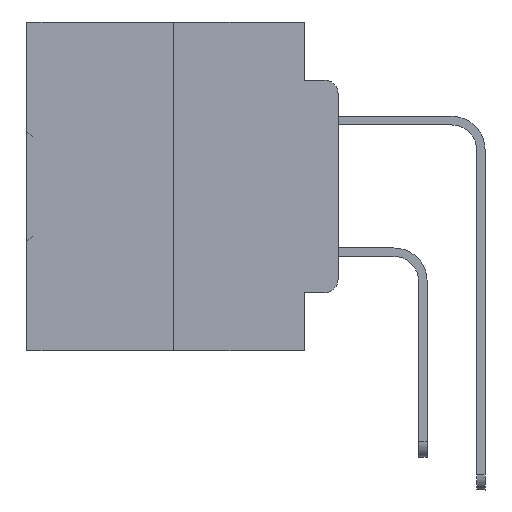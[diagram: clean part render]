
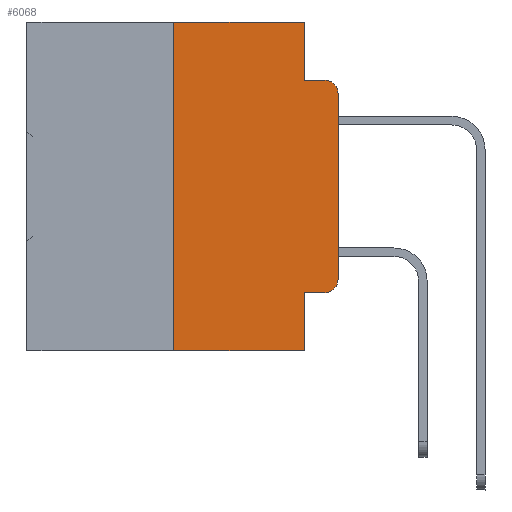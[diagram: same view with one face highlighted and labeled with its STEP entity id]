
A CAD part, left-side view. The second image highlights one B-rep face of the part: STEP entity #6068.
In plain terms, the highlighted planar face has unit normal (-1, 0, 0).
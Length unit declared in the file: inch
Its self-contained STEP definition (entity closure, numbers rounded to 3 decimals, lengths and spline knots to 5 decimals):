
#36 = ORIENTED_EDGE ( 'NONE', *, *, #22810, .F. ) ;
#89 = VECTOR ( 'NONE', #27309, 39.37008 ) ;
#466 = ORIENTED_EDGE ( 'NONE', *, *, #15825, .T. ) ;
#663 = DIRECTION ( 'NONE',  ( 0., -1., 0. ) ) ;
#906 = DIRECTION ( 'NONE',  ( 0., 0., 1. ) ) ;
#1231 = VERTEX_POINT ( 'NONE', #10744 ) ;
#1552 = CIRCLE ( 'NONE', #6538, 0.02 ) ;
#1707 = DIRECTION ( 'NONE',  ( 0., -1., 0. ) ) ;
#2793 = PLANE ( 'NONE',  #28297 ) ;
#3289 = VERTEX_POINT ( 'NONE', #22369 ) ;
#3346 = VERTEX_POINT ( 'NONE', #16937 ) ;
#3706 = EDGE_CURVE ( 'NONE', #19397, #1231, #22137, .T. ) ;
#4393 = CARTESIAN_POINT ( 'NONE',  ( 0., 0., -0.1085 ) ) ;
#5710 = DIRECTION ( 'NONE',  ( 0., 0., -1. ) ) ;
#6043 = EDGE_CURVE ( 'NONE', #19520, #1231, #1552, .T. ) ;
#6068 = ADVANCED_FACE ( 'NONE', ( #23015 ), #2793, .F. ) ;
#6453 = CARTESIAN_POINT ( 'NONE',  ( 0., 0.051, 0. ) ) ;
#6538 = AXIS2_PLACEMENT_3D ( 'NONE', #23588, #22820, #5710 ) ;
#6706 = AXIS2_PLACEMENT_3D ( 'NONE', #33310, #6827, #21218 ) ;
#6827 = DIRECTION ( 'NONE',  ( -1., 0., 0. ) ) ;
#6856 = LINE ( 'NONE', #18724, #20989 ) ;
#6894 = EDGE_LOOP ( 'NONE', ( #20061, #29721, #15955, #14135, #18119, #36357, #16792, #36, #466, #9473 ) ) ;
#7526 = LINE ( 'NONE', #15896, #27711 ) ;
#8056 = CARTESIAN_POINT ( 'NONE',  ( 0., 0.473, 0. ) ) ;
#8742 = VECTOR ( 'NONE', #31503, 39.37008 ) ;
#9473 = ORIENTED_EDGE ( 'NONE', *, *, #30266, .T. ) ;
#10744 = CARTESIAN_POINT ( 'NONE',  ( 0., 0.02, -0.0885 ) ) ;
#12270 = LINE ( 'NONE', #6453, #15726 ) ;
#12932 = CARTESIAN_POINT ( 'NONE',  ( 0., 0., -0.3915 ) ) ;
#13341 = VECTOR ( 'NONE', #663, 39.37008 ) ;
#14075 = DIRECTION ( 'NONE',  ( 1., 0., 0. ) ) ;
#14135 = ORIENTED_EDGE ( 'NONE', *, *, #27600, .F. ) ;
#15726 = VECTOR ( 'NONE', #17947, 39.37008 ) ;
#15825 = EDGE_CURVE ( 'NONE', #3289, #36625, #21860, .T. ) ;
#15896 = CARTESIAN_POINT ( 'NONE',  ( 0., 0., 0. ) ) ;
#15955 = ORIENTED_EDGE ( 'NONE', *, *, #3706, .F. ) ;
#16101 = CARTESIAN_POINT ( 'NONE',  ( 0., 0.051, 0. ) ) ;
#16626 = EDGE_CURVE ( 'NONE', #20588, #19520, #7526, .T. ) ;
#16792 = ORIENTED_EDGE ( 'NONE', *, *, #18825, .T. ) ;
#16937 = CARTESIAN_POINT ( 'NONE',  ( 0., 0.25, -0.5 ) ) ;
#17003 = DIRECTION ( 'NONE',  ( 0., 0., -1. ) ) ;
#17947 = DIRECTION ( 'NONE',  ( 0., 0., -1. ) ) ;
#18119 = ORIENTED_EDGE ( 'NONE', *, *, #23334, .F. ) ;
#18724 = CARTESIAN_POINT ( 'NONE',  ( 0., 0.473, -0.5 ) ) ;
#18825 = EDGE_CURVE ( 'NONE', #3346, #19817, #6856, .T. ) ;
#18917 = VECTOR ( 'NONE', #1707, 39.37008 ) ;
#19397 = VERTEX_POINT ( 'NONE', #36969 ) ;
#19520 = VERTEX_POINT ( 'NONE', #4393 ) ;
#19817 = VERTEX_POINT ( 'NONE', #25521 ) ;
#20061 = ORIENTED_EDGE ( 'NONE', *, *, #16626, .T. ) ;
#20071 = VERTEX_POINT ( 'NONE', #27407 ) ;
#20588 = VERTEX_POINT ( 'NONE', #12932 ) ;
#20989 = VECTOR ( 'NONE', #36254, 39.37008 ) ;
#21218 = DIRECTION ( 'NONE',  ( 0., 0., -1. ) ) ;
#21421 = DIRECTION ( 'NONE',  ( 0., 0., -1. ) ) ;
#21860 = LINE ( 'NONE', #33574, #13341 ) ;
#22137 = LINE ( 'NONE', #37535, #18917 ) ;
#22369 = CARTESIAN_POINT ( 'NONE',  ( 0., 0.051, -0.4115 ) ) ;
#22709 = CARTESIAN_POINT ( 'NONE',  ( 0., 0.473, 0. ) ) ;
#22810 = EDGE_CURVE ( 'NONE', #3289, #19817, #33130, .T. ) ;
#22820 = DIRECTION ( 'NONE',  ( -1., 0., 0. ) ) ;
#23015 = FACE_OUTER_BOUND ( 'NONE', #6894, .T. ) ;
#23334 = EDGE_CURVE ( 'NONE', #20071, #28018, #36952, .T. ) ;
#23470 = CIRCLE ( 'NONE', #6706, 0.02 ) ;
#23588 = CARTESIAN_POINT ( 'NONE',  ( 0., 0.02, -0.1085 ) ) ;
#24517 = CARTESIAN_POINT ( 'NONE',  ( 0., 0.051, 0. ) ) ;
#24554 = LINE ( 'NONE', #35889, #89 ) ;
#25521 = CARTESIAN_POINT ( 'NONE',  ( 0., 0.051, -0.5 ) ) ;
#25838 = EDGE_CURVE ( 'NONE', #3346, #20071, #24554, .T. ) ;
#27309 = DIRECTION ( 'NONE',  ( 0., 0., 1. ) ) ;
#27407 = CARTESIAN_POINT ( 'NONE',  ( 0., 0.25, 0. ) ) ;
#27600 = EDGE_CURVE ( 'NONE', #28018, #19397, #12270, .T. ) ;
#27711 = VECTOR ( 'NONE', #906, 39.37008 ) ;
#28018 = VERTEX_POINT ( 'NONE', #16101 ) ;
#28297 = AXIS2_PLACEMENT_3D ( 'NONE', #8056, #14075, #17003 ) ;
#29721 = ORIENTED_EDGE ( 'NONE', *, *, #6043, .T. ) ;
#29812 = CARTESIAN_POINT ( 'NONE',  ( 0., 0.02, -0.4115 ) ) ;
#30266 = EDGE_CURVE ( 'NONE', #36625, #20588, #23470, .T. ) ;
#31503 = DIRECTION ( 'NONE',  ( 0., -1., 0. ) ) ;
#33130 = LINE ( 'NONE', #24517, #34239 ) ;
#33310 = CARTESIAN_POINT ( 'NONE',  ( 0., 0.02, -0.3915 ) ) ;
#33574 = CARTESIAN_POINT ( 'NONE',  ( 0., 0.051, -0.4115 ) ) ;
#34239 = VECTOR ( 'NONE', #21421, 39.37008 ) ;
#35889 = CARTESIAN_POINT ( 'NONE',  ( 0., 0.25, 0. ) ) ;
#36254 = DIRECTION ( 'NONE',  ( 0., -1., 0. ) ) ;
#36357 = ORIENTED_EDGE ( 'NONE', *, *, #25838, .F. ) ;
#36625 = VERTEX_POINT ( 'NONE', #29812 ) ;
#36952 = LINE ( 'NONE', #22709, #8742 ) ;
#36969 = CARTESIAN_POINT ( 'NONE',  ( 0., 0.051, -0.0885 ) ) ;
#37535 = CARTESIAN_POINT ( 'NONE',  ( 0., 0.051, -0.0885 ) ) ;
